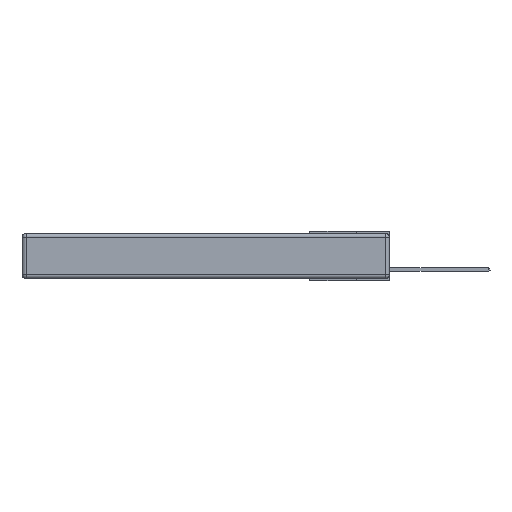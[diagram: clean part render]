
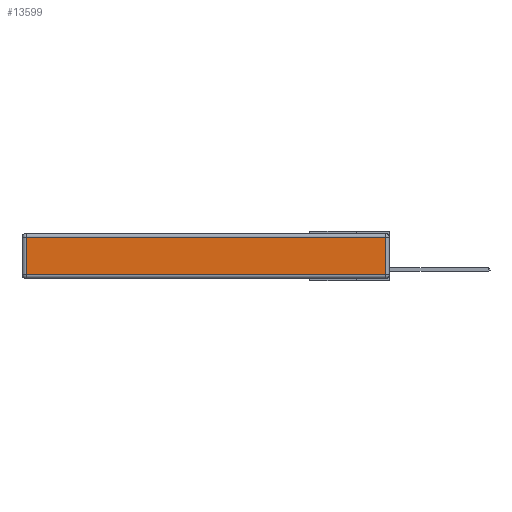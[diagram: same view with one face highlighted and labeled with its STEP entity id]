
A CAD part, left-side view. The second image highlights one B-rep face of the part: STEP entity #13599.
In plain terms, the highlighted planar face has unit normal (-1, 0, 0).
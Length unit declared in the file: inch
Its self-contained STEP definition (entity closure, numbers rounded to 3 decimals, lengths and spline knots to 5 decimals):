
#795 = CARTESIAN_POINT ( 'NONE',  ( 0., 0., -0.313 ) ) ;
#1432 = CARTESIAN_POINT ( 'NONE',  ( 0., 2.72, -0.03 ) ) ;
#1747 = ORIENTED_EDGE ( 'NONE', *, *, #2440, .T. ) ;
#1755 = LINE ( 'NONE', #795, #16131 ) ;
#2440 = EDGE_CURVE ( 'NONE', #2949, #11870, #11959, .T. ) ;
#2474 = CARTESIAN_POINT ( 'NONE',  ( 0., 2.72, -0.343 ) ) ;
#2949 = VERTEX_POINT ( 'NONE', #16583 ) ;
#3009 = LINE ( 'NONE', #9421, #11084 ) ;
#3979 = CARTESIAN_POINT ( 'NONE',  ( 0., 2.75, -0.03 ) ) ;
#4435 = CARTESIAN_POINT ( 'NONE',  ( 0., 2.72, -0.313 ) ) ;
#5506 = EDGE_LOOP ( 'NONE', ( #11750, #11113, #1747, #9447 ) ) ;
#6326 = VECTOR ( 'NONE', #9401, 39.37008 ) ;
#7465 = DIRECTION ( 'NONE',  ( 0., 0., 1. ) ) ;
#7527 = DIRECTION ( 'NONE',  ( -1., 0., 0. ) ) ;
#7573 = DIRECTION ( 'NONE',  ( 0., -1., 0. ) ) ;
#9124 = PLANE ( 'NONE',  #9282 ) ;
#9282 = AXIS2_PLACEMENT_3D ( 'NONE', #11888, #7527, #7465 ) ;
#9369 = DIRECTION ( 'NONE',  ( 0., 1., 0. ) ) ;
#9401 = DIRECTION ( 'NONE',  ( 0., 0., -1. ) ) ;
#9421 = CARTESIAN_POINT ( 'NONE',  ( 0., 0.03, -0.343 ) ) ;
#9447 = ORIENTED_EDGE ( 'NONE', *, *, #12056, .T. ) ;
#9764 = CARTESIAN_POINT ( 'NONE',  ( 0., 0.03, -0.313 ) ) ;
#9836 = VECTOR ( 'NONE', #9369, 39.37008 ) ;
#11084 = VECTOR ( 'NONE', #17614, 39.37008 ) ;
#11113 = ORIENTED_EDGE ( 'NONE', *, *, #13220, .T. ) ;
#11750 = ORIENTED_EDGE ( 'NONE', *, *, #17527, .T. ) ;
#11870 = VERTEX_POINT ( 'NONE', #1432 ) ;
#11888 = CARTESIAN_POINT ( 'NONE',  ( 0., 0., -0.343 ) ) ;
#11959 = LINE ( 'NONE', #3979, #9836 ) ;
#12056 = EDGE_CURVE ( 'NONE', #11870, #17974, #16748, .T. ) ;
#12597 = FACE_OUTER_BOUND ( 'NONE', #5506, .T. ) ;
#13220 = EDGE_CURVE ( 'NONE', #17235, #2949, #3009, .T. ) ;
#13599 = ADVANCED_FACE ( 'NONE', ( #12597 ), #9124, .T. ) ;
#16131 = VECTOR ( 'NONE', #7573, 39.37008 ) ;
#16583 = CARTESIAN_POINT ( 'NONE',  ( 0., 0.03, -0.03 ) ) ;
#16748 = LINE ( 'NONE', #2474, #6326 ) ;
#17235 = VERTEX_POINT ( 'NONE', #9764 ) ;
#17527 = EDGE_CURVE ( 'NONE', #17974, #17235, #1755, .T. ) ;
#17614 = DIRECTION ( 'NONE',  ( 0., 0., 1. ) ) ;
#17974 = VERTEX_POINT ( 'NONE', #4435 ) ;
